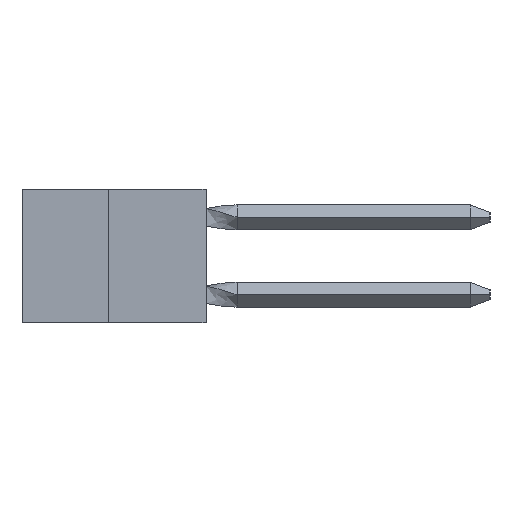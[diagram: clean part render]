
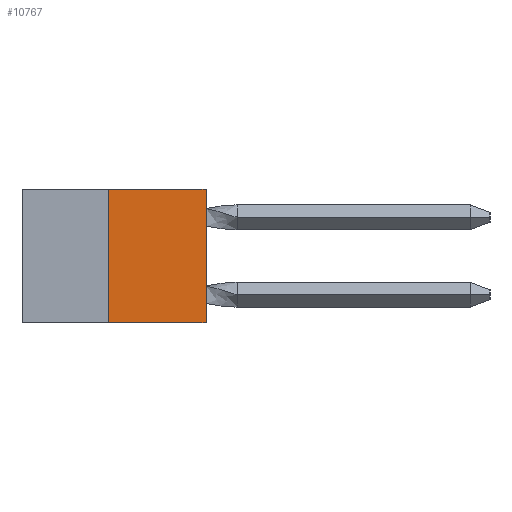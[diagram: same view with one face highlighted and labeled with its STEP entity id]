
A CAD part, left-side view. The second image highlights one B-rep face of the part: STEP entity #10767.
In plain terms, the highlighted planar face has unit normal (-1, 0, 0).
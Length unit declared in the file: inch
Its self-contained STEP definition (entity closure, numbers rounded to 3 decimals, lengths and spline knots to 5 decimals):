
#1565 = PLANE ( 'NONE',  #30390 ) ;
#5034 = CARTESIAN_POINT ( 'NONE',  ( 0., 0.473, 0. ) ) ;
#6837 = LINE ( 'NONE', #20087, #20890 ) ;
#8193 = LINE ( 'NONE', #10429, #9818 ) ;
#9818 = VECTOR ( 'NONE', #10879, 39.37008 ) ;
#10429 = CARTESIAN_POINT ( 'NONE',  ( 0., 0., 0. ) ) ;
#10767 = ADVANCED_FACE ( 'NONE', ( #18849 ), #1565, .F. ) ;
#10879 = DIRECTION ( 'NONE',  ( 0., 0., 1. ) ) ;
#12810 = ORIENTED_EDGE ( 'NONE', *, *, #33352, .F. ) ;
#14056 = CARTESIAN_POINT ( 'NONE',  ( 0., 0., -0.343 ) ) ;
#15460 = VERTEX_POINT ( 'NONE', #30641 ) ;
#16863 = LINE ( 'NONE', #23846, #35378 ) ;
#18528 = CARTESIAN_POINT ( 'NONE',  ( 0., 0.473, -0.343 ) ) ;
#18749 = ORIENTED_EDGE ( 'NONE', *, *, #39387, .T. ) ;
#18849 = FACE_OUTER_BOUND ( 'NONE', #22381, .T. ) ;
#19218 = DIRECTION ( 'NONE',  ( 0., 0., -1. ) ) ;
#20087 = CARTESIAN_POINT ( 'NONE',  ( 0., 0.25, 0. ) ) ;
#20550 = EDGE_CURVE ( 'NONE', #15460, #34633, #16863, .T. ) ;
#20724 = ORIENTED_EDGE ( 'NONE', *, *, #36820, .T. ) ;
#20890 = VECTOR ( 'NONE', #23456, 39.37008 ) ;
#22381 = EDGE_LOOP ( 'NONE', ( #32836, #12810, #20724, #18749 ) ) ;
#23456 = DIRECTION ( 'NONE',  ( 0., 0., 1. ) ) ;
#23632 = CARTESIAN_POINT ( 'NONE',  ( 0., 0.25, -0.343 ) ) ;
#23846 = CARTESIAN_POINT ( 'NONE',  ( 0., 0.473, 0. ) ) ;
#24156 = DIRECTION ( 'NONE',  ( 0., -1., 0. ) ) ;
#24438 = VERTEX_POINT ( 'NONE', #23632 ) ;
#25240 = VECTOR ( 'NONE', #42821, 39.37008 ) ;
#30390 = AXIS2_PLACEMENT_3D ( 'NONE', #5034, #43235, #19218 ) ;
#30641 = CARTESIAN_POINT ( 'NONE',  ( 0., 0.25, 0. ) ) ;
#32836 = ORIENTED_EDGE ( 'NONE', *, *, #20550, .F. ) ;
#32917 = VERTEX_POINT ( 'NONE', #14056 ) ;
#33352 = EDGE_CURVE ( 'NONE', #24438, #15460, #6837, .T. ) ;
#34633 = VERTEX_POINT ( 'NONE', #37123 ) ;
#35378 = VECTOR ( 'NONE', #24156, 39.37008 ) ;
#36820 = EDGE_CURVE ( 'NONE', #24438, #32917, #43681, .T. ) ;
#37123 = CARTESIAN_POINT ( 'NONE',  ( 0., 0., 0. ) ) ;
#39387 = EDGE_CURVE ( 'NONE', #32917, #34633, #8193, .T. ) ;
#42821 = DIRECTION ( 'NONE',  ( 0., -1., 0. ) ) ;
#43235 = DIRECTION ( 'NONE',  ( 1., 0., 0. ) ) ;
#43681 = LINE ( 'NONE', #18528, #25240 ) ;
